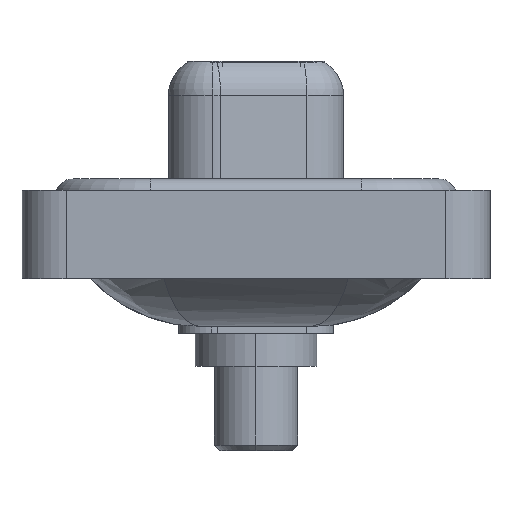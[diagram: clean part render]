
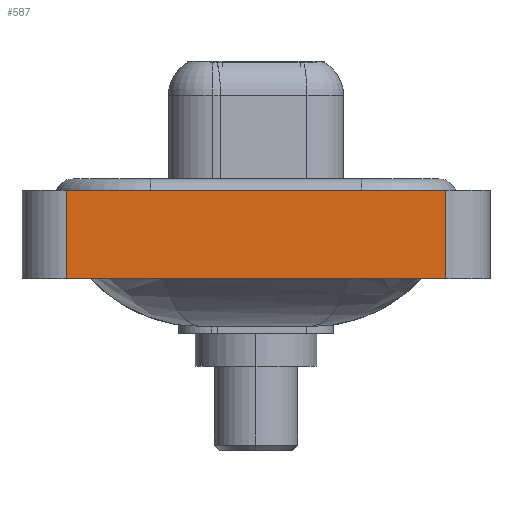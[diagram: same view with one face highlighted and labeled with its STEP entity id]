
A CAD part, left-side view. The second image highlights one B-rep face of the part: STEP entity #587.
In plain terms, the highlighted planar face has unit normal (-1, 0, 0).
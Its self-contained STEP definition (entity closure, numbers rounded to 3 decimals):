
#126 = CARTESIAN_POINT ( 'NONE',  ( -7.35, -8.55, 0.4 ) ) ;
#328 = DIRECTION ( 'NONE',  ( 0., -1., 0. ) ) ;
#554 = CARTESIAN_POINT ( 'NONE',  ( -7.35, 8.55, -3.6 ) ) ;
#587 = ADVANCED_FACE ( 'NONE', ( #14917 ), #3261, .T. ) ;
#1219 = LINE ( 'NONE', #11631, #9088 ) ;
#1864 = ORIENTED_EDGE ( 'NONE', *, *, #8097, .T. ) ;
#2009 = DIRECTION ( 'NONE',  ( 0., 0., 1. ) ) ;
#2126 = LINE ( 'NONE', #8398, #3911 ) ;
#2162 = ORIENTED_EDGE ( 'NONE', *, *, #15697, .T. ) ;
#3261 = PLANE ( 'NONE',  #7120 ) ;
#3417 = VERTEX_POINT ( 'NONE', #15924 ) ;
#3911 = VECTOR ( 'NONE', #13457, 1000. ) ;
#4007 = ORIENTED_EDGE ( 'NONE', *, *, #6172, .F. ) ;
#4250 = DIRECTION ( 'NONE',  ( 0., -1., 0. ) ) ;
#5123 = CARTESIAN_POINT ( 'NONE',  ( -7.35, 8.55, -3.6 ) ) ;
#5410 = VERTEX_POINT ( 'NONE', #12135 ) ;
#5423 = ORIENTED_EDGE ( 'NONE', *, *, #11311, .F. ) ;
#6172 = EDGE_CURVE ( 'NONE', #3417, #8403, #1219, .T. ) ;
#6809 = DIRECTION ( 'NONE',  ( 0., 0., 1. ) ) ;
#6865 = EDGE_LOOP ( 'NONE', ( #2162, #4007, #5423, #1864 ) ) ;
#7120 = AXIS2_PLACEMENT_3D ( 'NONE', #8288, #13346, #2009 ) ;
#8097 = EDGE_CURVE ( 'NONE', #14186, #5410, #8218, .T. ) ;
#8218 = LINE ( 'NONE', #15586, #11785 ) ;
#8288 = CARTESIAN_POINT ( 'NONE',  ( -7.35, -8.55, -3.6 ) ) ;
#8398 = CARTESIAN_POINT ( 'NONE',  ( -7.35, -8.55, -3.6 ) ) ;
#8403 = VERTEX_POINT ( 'NONE', #126 ) ;
#9088 = VECTOR ( 'NONE', #328, 1000. ) ;
#10630 = VECTOR ( 'NONE', #6809, 1000. ) ;
#11311 = EDGE_CURVE ( 'NONE', #14186, #3417, #13186, .T. ) ;
#11631 = CARTESIAN_POINT ( 'NONE',  ( -7.35, -8.55, 0.4 ) ) ;
#11785 = VECTOR ( 'NONE', #4250, 1000. ) ;
#12135 = CARTESIAN_POINT ( 'NONE',  ( -7.35, -8.55, -3.6 ) ) ;
#13186 = LINE ( 'NONE', #554, #10630 ) ;
#13346 = DIRECTION ( 'NONE',  ( -1., 0., 0. ) ) ;
#13457 = DIRECTION ( 'NONE',  ( 0., 0., 1. ) ) ;
#14186 = VERTEX_POINT ( 'NONE', #5123 ) ;
#14917 = FACE_OUTER_BOUND ( 'NONE', #6865, .T. ) ;
#15586 = CARTESIAN_POINT ( 'NONE',  ( -7.35, -8.55, -3.6 ) ) ;
#15697 = EDGE_CURVE ( 'NONE', #5410, #8403, #2126, .T. ) ;
#15924 = CARTESIAN_POINT ( 'NONE',  ( -7.35, 8.55, 0.4 ) ) ;
